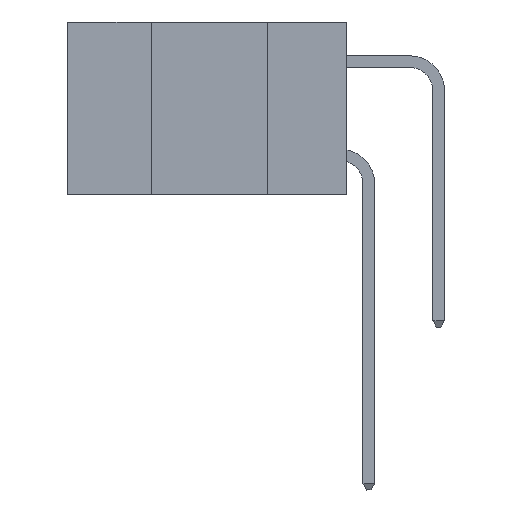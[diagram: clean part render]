
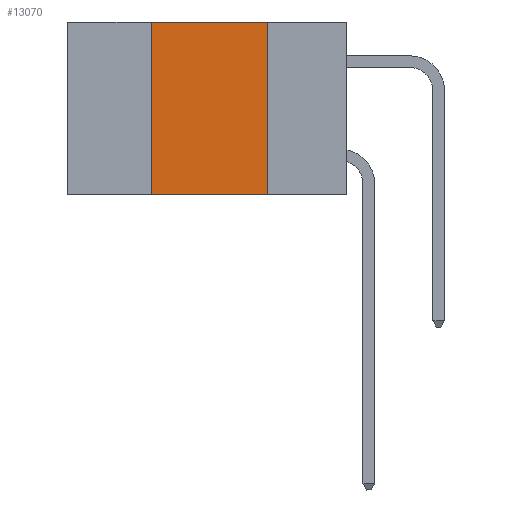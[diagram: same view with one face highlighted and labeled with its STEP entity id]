
A CAD part, left-side view. The second image highlights one B-rep face of the part: STEP entity #13070.
In plain terms, the highlighted planar face has unit normal (-1, 0, 0).
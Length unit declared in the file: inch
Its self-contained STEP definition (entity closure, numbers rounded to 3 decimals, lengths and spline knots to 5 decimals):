
#1146 = DIRECTION ( 'NONE',  ( 0., -1., 0. ) ) ;
#1672 = FACE_OUTER_BOUND ( 'NONE', #6303, .T. ) ;
#1944 = CARTESIAN_POINT ( 'NONE',  ( 0., 0.42, 0. ) ) ;
#3183 = CARTESIAN_POINT ( 'NONE',  ( 0., 0.42, -0.37 ) ) ;
#3533 = VERTEX_POINT ( 'NONE', #14644 ) ;
#4171 = CARTESIAN_POINT ( 'NONE',  ( 0., 0.6, -0.37 ) ) ;
#6303 = EDGE_LOOP ( 'NONE', ( #6614, #35019, #31176, #29177 ) ) ;
#6614 = ORIENTED_EDGE ( 'NONE', *, *, #37537, .F. ) ;
#8299 = DIRECTION ( 'NONE',  ( 0., 0., -1. ) ) ;
#9443 = CARTESIAN_POINT ( 'NONE',  ( 0., 0.42, 0. ) ) ;
#10428 = AXIS2_PLACEMENT_3D ( 'NONE', #20415, #38878, #8299 ) ;
#10657 = VERTEX_POINT ( 'NONE', #3183 ) ;
#11947 = VECTOR ( 'NONE', #19478, 39.37008 ) ;
#12087 = VECTOR ( 'NONE', #24401, 39.37008 ) ;
#13070 = ADVANCED_FACE ( 'NONE', ( #1672 ), #32469, .F. ) ;
#14644 = CARTESIAN_POINT ( 'NONE',  ( 0., 0.17, 0. ) ) ;
#15376 = CARTESIAN_POINT ( 'NONE',  ( 0., 0.17, -0.37 ) ) ;
#19478 = DIRECTION ( 'NONE',  ( 0., -1., 0. ) ) ;
#19663 = VERTEX_POINT ( 'NONE', #15376 ) ;
#20075 = CARTESIAN_POINT ( 'NONE',  ( 0., 0.6, 0. ) ) ;
#20415 = CARTESIAN_POINT ( 'NONE',  ( 0., 0.6, 0. ) ) ;
#21781 = EDGE_CURVE ( 'NONE', #10657, #25995, #33996, .T. ) ;
#24062 = VECTOR ( 'NONE', #1146, 39.37008 ) ;
#24401 = DIRECTION ( 'NONE',  ( 0., 0., -1. ) ) ;
#25708 = LINE ( 'NONE', #4171, #24062 ) ;
#25995 = VERTEX_POINT ( 'NONE', #1944 ) ;
#26746 = EDGE_CURVE ( 'NONE', #10657, #19663, #25708, .T. ) ;
#27226 = CARTESIAN_POINT ( 'NONE',  ( 0., 0.17, 0. ) ) ;
#29177 = ORIENTED_EDGE ( 'NONE', *, *, #26746, .T. ) ;
#29310 = LINE ( 'NONE', #20075, #11947 ) ;
#30279 = VECTOR ( 'NONE', #36812, 39.37008 ) ;
#31176 = ORIENTED_EDGE ( 'NONE', *, *, #21781, .F. ) ;
#32469 = PLANE ( 'NONE',  #10428 ) ;
#33996 = LINE ( 'NONE', #9443, #30279 ) ;
#35019 = ORIENTED_EDGE ( 'NONE', *, *, #35076, .F. ) ;
#35076 = EDGE_CURVE ( 'NONE', #25995, #3533, #29310, .T. ) ;
#36812 = DIRECTION ( 'NONE',  ( 0., 0., 1. ) ) ;
#37537 = EDGE_CURVE ( 'NONE', #3533, #19663, #39655, .T. ) ;
#38878 = DIRECTION ( 'NONE',  ( 1., 0., 0. ) ) ;
#39655 = LINE ( 'NONE', #27226, #12087 ) ;
